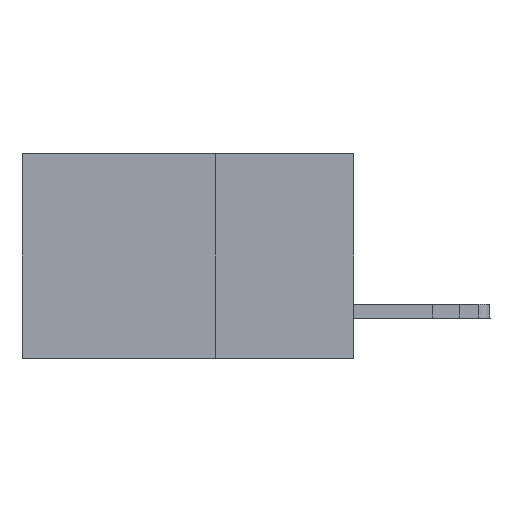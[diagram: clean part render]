
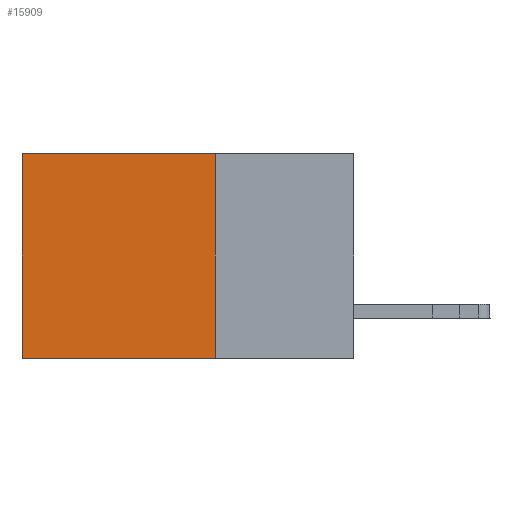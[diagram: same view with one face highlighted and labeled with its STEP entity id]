
A CAD part, left-side view. The second image highlights one B-rep face of the part: STEP entity #15909.
In plain terms, the highlighted planar face has unit normal (-1, 0, 0).
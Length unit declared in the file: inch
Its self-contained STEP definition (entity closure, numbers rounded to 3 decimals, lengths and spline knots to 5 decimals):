
#922 = VECTOR ( 'NONE', #4648, 39.37008 ) ;
#2368 = ORIENTED_EDGE ( 'NONE', *, *, #16049, .T. ) ;
#4042 = CARTESIAN_POINT ( 'NONE',  ( 0.2875, 0.25, -0.37 ) ) ;
#4287 = EDGE_CURVE ( 'NONE', #18872, #15239, #21489, .T. ) ;
#4648 = DIRECTION ( 'NONE',  ( 0., 0., -1. ) ) ;
#4877 = EDGE_CURVE ( 'NONE', #16178, #15239, #16096, .T. ) ;
#5316 = AXIS2_PLACEMENT_3D ( 'NONE', #12029, #15603, #11916 ) ;
#5933 = CARTESIAN_POINT ( 'NONE',  ( 0.2875, 0.25, -0.37 ) ) ;
#6051 = EDGE_LOOP ( 'NONE', ( #12700, #10909, #13595, #2368 ) ) ;
#7589 = VECTOR ( 'NONE', #22498, 39.37008 ) ;
#8318 = LINE ( 'NONE', #10045, #7589 ) ;
#8562 = PLANE ( 'NONE',  #5316 ) ;
#8793 = DIRECTION ( 'NONE',  ( 0., 1., 0. ) ) ;
#9030 = VECTOR ( 'NONE', #8793, 39.37008 ) ;
#10045 = CARTESIAN_POINT ( 'NONE',  ( 0.2875, 0.25, 0. ) ) ;
#10909 = ORIENTED_EDGE ( 'NONE', *, *, #4287, .F. ) ;
#11916 = DIRECTION ( 'NONE',  ( 0., 0., -1. ) ) ;
#12029 = CARTESIAN_POINT ( 'NONE',  ( 0.2875, 0.25, 0. ) ) ;
#12700 = ORIENTED_EDGE ( 'NONE', *, *, #4877, .T. ) ;
#13595 = ORIENTED_EDGE ( 'NONE', *, *, #22173, .F. ) ;
#13830 = VERTEX_POINT ( 'NONE', #14834 ) ;
#14193 = LINE ( 'NONE', #16278, #9030 ) ;
#14834 = CARTESIAN_POINT ( 'NONE',  ( 0.2875, 0.25, 0. ) ) ;
#15239 = VERTEX_POINT ( 'NONE', #18074 ) ;
#15603 = DIRECTION ( 'NONE',  ( 1., 0., 0. ) ) ;
#15909 = ADVANCED_FACE ( 'NONE', ( #19176 ), #8562, .F. ) ;
#16049 = EDGE_CURVE ( 'NONE', #13830, #16178, #14193, .T. ) ;
#16096 = LINE ( 'NONE', #18734, #922 ) ;
#16123 = DIRECTION ( 'NONE',  ( 0., 1., 0. ) ) ;
#16178 = VERTEX_POINT ( 'NONE', #21532 ) ;
#16278 = CARTESIAN_POINT ( 'NONE',  ( 0.2875, 0.25, 0. ) ) ;
#16809 = VECTOR ( 'NONE', #16123, 39.37008 ) ;
#18074 = CARTESIAN_POINT ( 'NONE',  ( 0.2875, 0.6, -0.37 ) ) ;
#18734 = CARTESIAN_POINT ( 'NONE',  ( 0.2875, 0.6, 0. ) ) ;
#18872 = VERTEX_POINT ( 'NONE', #4042 ) ;
#19176 = FACE_OUTER_BOUND ( 'NONE', #6051, .T. ) ;
#21489 = LINE ( 'NONE', #5933, #16809 ) ;
#21532 = CARTESIAN_POINT ( 'NONE',  ( 0.2875, 0.6, 0. ) ) ;
#22173 = EDGE_CURVE ( 'NONE', #13830, #18872, #8318, .T. ) ;
#22498 = DIRECTION ( 'NONE',  ( 0., 0., -1. ) ) ;
